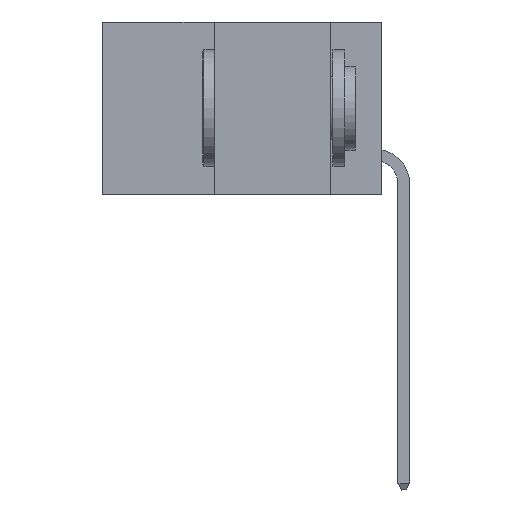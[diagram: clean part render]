
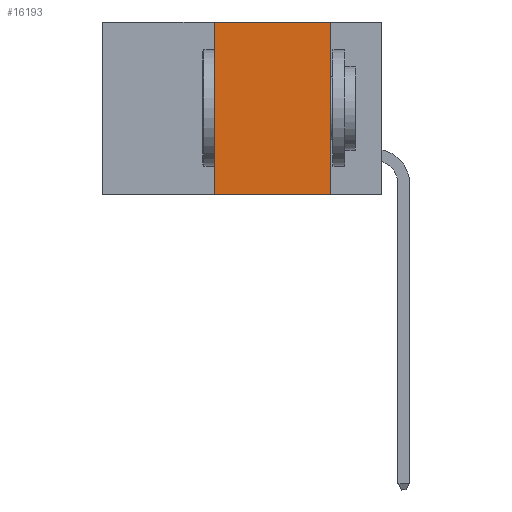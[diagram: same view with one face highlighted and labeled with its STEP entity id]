
A CAD part, left-side view. The second image highlights one B-rep face of the part: STEP entity #16193.
In plain terms, the highlighted planar face has unit normal (-1, 0, 0).
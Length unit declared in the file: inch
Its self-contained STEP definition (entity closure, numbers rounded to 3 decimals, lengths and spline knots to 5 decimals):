
#416 = CARTESIAN_POINT ( 'NONE',  ( 0., 0.6, 0. ) ) ;
#854 = DIRECTION ( 'NONE',  ( 0., 0., -1. ) ) ;
#3212 = VECTOR ( 'NONE', #14730, 39.37008 ) ;
#3229 = EDGE_CURVE ( 'NONE', #17430, #6241, #4305, .T. ) ;
#4305 = LINE ( 'NONE', #416, #3212 ) ;
#4950 = EDGE_LOOP ( 'NONE', ( #27074, #32409, #18512, #15441 ) ) ;
#6241 = VERTEX_POINT ( 'NONE', #37667 ) ;
#7047 = EDGE_CURVE ( 'NONE', #6241, #16114, #14782, .T. ) ;
#8154 = CARTESIAN_POINT ( 'NONE',  ( 0., 0.11, -0.37 ) ) ;
#8530 = AXIS2_PLACEMENT_3D ( 'NONE', #36678, #15377, #40194 ) ;
#11002 = DIRECTION ( 'NONE',  ( 0., -1., 0. ) ) ;
#11312 = CARTESIAN_POINT ( 'NONE',  ( 0., 0.6, -0.37 ) ) ;
#13626 = LINE ( 'NONE', #11312, #24074 ) ;
#14079 = CARTESIAN_POINT ( 'NONE',  ( 0., 0.36, 0. ) ) ;
#14730 = DIRECTION ( 'NONE',  ( 0., -1., 0. ) ) ;
#14736 = LINE ( 'NONE', #14079, #45395 ) ;
#14782 = LINE ( 'NONE', #21477, #30162 ) ;
#15377 = DIRECTION ( 'NONE',  ( 1., 0., 0. ) ) ;
#15441 = ORIENTED_EDGE ( 'NONE', *, *, #39671, .T. ) ;
#16114 = VERTEX_POINT ( 'NONE', #8154 ) ;
#16193 = ADVANCED_FACE ( 'NONE', ( #32928 ), #18895, .F. ) ;
#16896 = CARTESIAN_POINT ( 'NONE',  ( 0., 0.36, 0. ) ) ;
#17430 = VERTEX_POINT ( 'NONE', #16896 ) ;
#18512 = ORIENTED_EDGE ( 'NONE', *, *, #26093, .F. ) ;
#18895 = PLANE ( 'NONE',  #8530 ) ;
#20125 = VERTEX_POINT ( 'NONE', #26028 ) ;
#21477 = CARTESIAN_POINT ( 'NONE',  ( 0., 0.11, 0. ) ) ;
#24074 = VECTOR ( 'NONE', #11002, 39.37008 ) ;
#26028 = CARTESIAN_POINT ( 'NONE',  ( 0., 0.36, -0.37 ) ) ;
#26093 = EDGE_CURVE ( 'NONE', #20125, #17430, #14736, .T. ) ;
#27074 = ORIENTED_EDGE ( 'NONE', *, *, #7047, .F. ) ;
#30162 = VECTOR ( 'NONE', #854, 39.37008 ) ;
#31590 = DIRECTION ( 'NONE',  ( 0., 0., 1. ) ) ;
#32409 = ORIENTED_EDGE ( 'NONE', *, *, #3229, .F. ) ;
#32928 = FACE_OUTER_BOUND ( 'NONE', #4950, .T. ) ;
#36678 = CARTESIAN_POINT ( 'NONE',  ( 0., 0.6, 0. ) ) ;
#37667 = CARTESIAN_POINT ( 'NONE',  ( 0., 0.11, 0. ) ) ;
#39671 = EDGE_CURVE ( 'NONE', #20125, #16114, #13626, .T. ) ;
#40194 = DIRECTION ( 'NONE',  ( 0., 0., -1. ) ) ;
#45395 = VECTOR ( 'NONE', #31590, 39.37008 ) ;
